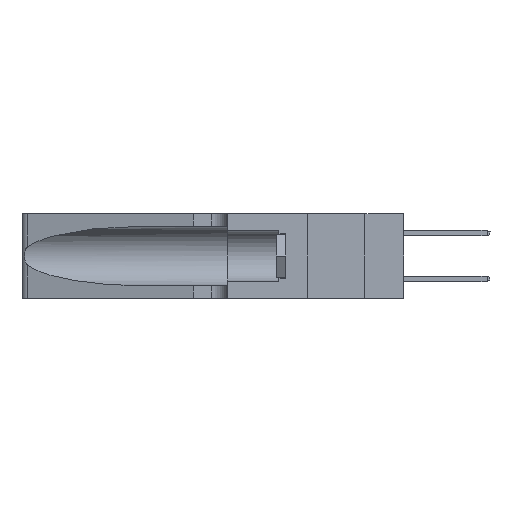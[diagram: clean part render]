
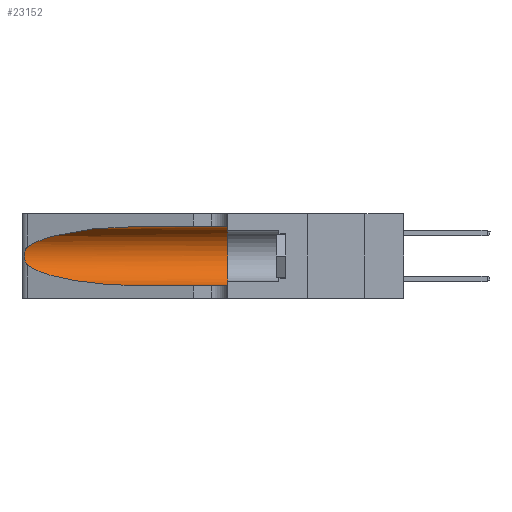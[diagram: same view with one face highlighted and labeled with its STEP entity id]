
A CAD part, left-side view. The second image highlights one B-rep face of the part: STEP entity #23152.
In plain terms, the highlighted cylindrical face has radius 3.308 mm (diameter 6.617 mm), a partial arc.
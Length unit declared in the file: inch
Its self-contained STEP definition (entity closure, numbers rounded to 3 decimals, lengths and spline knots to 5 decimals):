
#36 = CARTESIAN_POINT ( 'NONE',  ( 0.25487, 1.22718, 0.14631 ) ) ;
#103 = VERTEX_POINT ( 'NONE', #14063 ) ;
#513 = CARTESIAN_POINT ( 'NONE',  ( 0.25639, 1.23184, 0.21858 ) ) ;
#550 = VERTEX_POINT ( 'NONE', #15759 ) ;
#1061 = CARTESIAN_POINT ( 'NONE',  ( 0.25487, 1.22718, 0.22369 ) ) ;
#1993 = VERTEX_POINT ( 'NONE', #6420 ) ;
#2112 = CARTESIAN_POINT ( 'NONE',  ( 0.2373, 1.15595, 0.28018 ) ) ;
#2521 = CARTESIAN_POINT ( 'NONE',  ( 0.25854, 1.2359, 0.20912 ) ) ;
#3727 = CARTESIAN_POINT ( 'NONE',  ( 0.1305, 0.35, 0.185 ) ) ;
#3880 = LINE ( 'NONE', #5275, #13383 ) ;
#4057 = ORIENTED_EDGE ( 'NONE', *, *, #11811, .F. ) ;
#4451 = CARTESIAN_POINT ( 'NONE',  ( 0.26075, 1.23896, 0.19203 ) ) ;
#5275 = CARTESIAN_POINT ( 'NONE',  ( 0.1305, 1.61858, 0.05475 ) ) ;
#5277 = ORIENTED_EDGE ( 'NONE', *, *, #23271, .F. ) ;
#5668 = DIRECTION ( 'NONE',  ( 0., 0., 1. ) ) ;
#5710 = FACE_OUTER_BOUND ( 'NONE', #21056, .T. ) ;
#6384 = CARTESIAN_POINT ( 'NONE',  ( 0.26017, 1.23833, 0.17102 ) ) ;
#6420 = CARTESIAN_POINT ( 'NONE',  ( 0.1305, 0.72297, 0.31525 ) ) ;
#6728 = ORIENTED_EDGE ( 'NONE', *, *, #9442, .T. ) ;
#6790 = DIRECTION ( 'NONE',  ( 0., 0., -1. ) ) ;
#6835 = CARTESIAN_POINT ( 'NONE',  ( 0.2373, 1.15595, 0.08982 ) ) ;
#7212 = CARTESIAN_POINT ( 'NONE',  ( 0.1305, 0.72297, 0.05475 ) ) ;
#7220 = CARTESIAN_POINT ( 'NONE',  ( 0.1305, 1.61858, 0.31525 ) ) ;
#7690 = VERTEX_POINT ( 'NONE', #7212 ) ;
#7900 = VERTEX_POINT ( 'NONE', #36 ) ;
#8309 = CARTESIAN_POINT ( 'NONE',  ( 0.25789, 1.23486, 0.15765 ) ) ;
#8781 = CARTESIAN_POINT ( 'NONE',  ( 0.25487, 1.22718, 0.14631 ) ) ;
#9150 = DIRECTION ( 'NONE',  ( 0., -1., 0. ) ) ;
#9442 = EDGE_CURVE ( 'NONE', #15122, #7900, #23073, .T. ) ;
#10155 = CARTESIAN_POINT ( 'NONE',  ( 0.25487, 1.22718, 0.22369 ) ) ;
#10236 = CARTESIAN_POINT ( 'NONE',  ( 0.25555, 1.22993, 0.14849 ) ) ;
#10695 = CARTESIAN_POINT ( 'NONE',  ( 0.18966, 0.96281, 0.05475 ) ) ;
#11023 = EDGE_CURVE ( 'NONE', #7900, #7690, #14643, .T. ) ;
#11635 = CARTESIAN_POINT ( 'NONE',  ( 0.1305, 0.72297, 0.31525 ) ) ;
#11811 = EDGE_CURVE ( 'NONE', #550, #103, #18386, .T. ) ;
#12042 = CARTESIAN_POINT ( 'NONE',  ( 0.25555, 1.22994, 0.2215 ) ) ;
#13383 = VECTOR ( 'NONE', #18305, 39.37008 ) ;
#13912 = CARTESIAN_POINT ( 'NONE',  ( 0.25787, 1.23484, 0.2124 ) ) ;
#14049 = AXIS2_PLACEMENT_3D ( 'NONE', #3727, #16869, #5668 ) ;
#14063 = CARTESIAN_POINT ( 'NONE',  ( 0.1305, 0.35, 0.05475 ) ) ;
#14317 = DIRECTION ( 'NONE',  ( 0., -1., 0. ) ) ;
#14417 = ORIENTED_EDGE ( 'NONE', *, *, #20048, .T. ) ;
#14643 =( BOUNDED_CURVE ( )  B_SPLINE_CURVE ( 3, ( #8781, #6835, #10695, #23467 ),
 .UNSPECIFIED., .F., .F. ) 
 B_SPLINE_CURVE_WITH_KNOTS ( ( 4, 4 ),
 ( 3.44316, 4.71239 ),
 .UNSPECIFIED. ) 
 CURVE ( )  GEOMETRIC_REPRESENTATION_ITEM ( )  RATIONAL_B_SPLINE_CURVE ( ( 1., 0.87, 0.87, 1. ) ) 
 REPRESENTATION_ITEM ( '' )  );
#15110 = CYLINDRICAL_SURFACE ( 'NONE', #16166, 0.13025 ) ;
#15122 = VERTEX_POINT ( 'NONE', #1061 ) ;
#15332 = CARTESIAN_POINT ( 'NONE',  ( 0.25487, 1.22718, 0.22369 ) ) ;
#15728 = CARTESIAN_POINT ( 'NONE',  ( 0.26018, 1.23835, 0.19895 ) ) ;
#15759 = CARTESIAN_POINT ( 'NONE',  ( 0.1305, 0.35, 0.31525 ) ) ;
#16122 = CARTESIAN_POINT ( 'NONE',  ( 0.1305, 1.61858, 0.185 ) ) ;
#16166 = AXIS2_PLACEMENT_3D ( 'NONE', #16122, #14317, #6790 ) ;
#16869 = DIRECTION ( 'NONE',  ( 0., 1., 0. ) ) ;
#17257 = ORIENTED_EDGE ( 'NONE', *, *, #11023, .T. ) ;
#17552 = CARTESIAN_POINT ( 'NONE',  ( 0.26075, 1.23896, 0.178 ) ) ;
#18305 = DIRECTION ( 'NONE',  ( 0., -1., 0. ) ) ;
#18386 = CIRCLE ( 'NONE', #14049, 0.13025 ) ;
#19354 = CARTESIAN_POINT ( 'NONE',  ( 0.25856, 1.23593, 0.16098 ) ) ;
#20048 = EDGE_CURVE ( 'NONE', #1993, #15122, #21308, .T. ) ;
#21056 = EDGE_LOOP ( 'NONE', ( #14417, #6728, #17257, #22643, #4057, #5277 ) ) ;
#21132 = EDGE_CURVE ( 'NONE', #7690, #103, #3880, .T. ) ;
#21183 = CARTESIAN_POINT ( 'NONE',  ( 0.25639, 1.23186, 0.15144 ) ) ;
#21308 =( BOUNDED_CURVE ( )  B_SPLINE_CURVE ( 3, ( #11635, #22557, #2112, #15332 ),
 .UNSPECIFIED., .F., .F. ) 
 B_SPLINE_CURVE_WITH_KNOTS ( ( 4, 4 ),
 ( 1.5708, 2.84003 ),
 .UNSPECIFIED. ) 
 CURVE ( )  GEOMETRIC_REPRESENTATION_ITEM ( )  RATIONAL_B_SPLINE_CURVE ( ( 1., 0.87, 0.87, 1. ) ) 
 REPRESENTATION_ITEM ( '' )  );
#21902 = VECTOR ( 'NONE', #9150, 39.37008 ) ;
#22479 = LINE ( 'NONE', #7220, #21902 ) ;
#22557 = CARTESIAN_POINT ( 'NONE',  ( 0.18966, 0.96281, 0.31525 ) ) ;
#22643 = ORIENTED_EDGE ( 'NONE', *, *, #21132, .T. ) ;
#23025 = CARTESIAN_POINT ( 'NONE',  ( 0.25487, 1.22718, 0.14631 ) ) ;
#23073 = B_SPLINE_CURVE_WITH_KNOTS ( 'NONE', 3,
 ( #10155, #12042, #513, #13912, #2521, #15728, #4451, #17552, #6384, #19354, #8309, #21183, #10236, #23025 ),
 .UNSPECIFIED., .F., .F.,
 ( 4, 2, 2, 2, 2, 2, 4 ),
 ( 0., 0.00027, 0.00053, 0.00107, 0.0016, 0.00187, 0.00214 ),
 .UNSPECIFIED. ) ;
#23152 = ADVANCED_FACE ( 'NONE', ( #5710 ), #15110, .F. ) ;
#23271 = EDGE_CURVE ( 'NONE', #1993, #550, #22479, .T. ) ;
#23467 = CARTESIAN_POINT ( 'NONE',  ( 0.1305, 0.72297, 0.05475 ) ) ;
